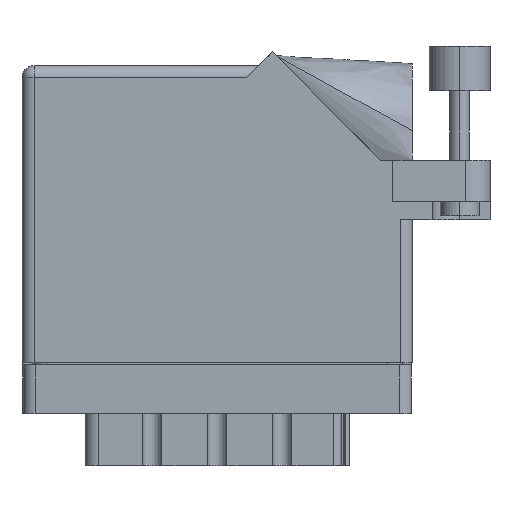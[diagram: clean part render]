
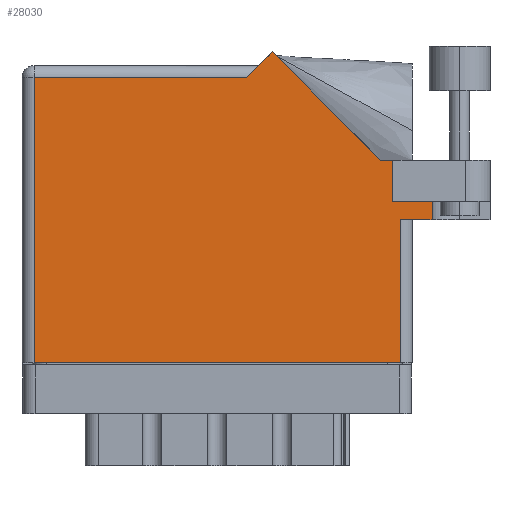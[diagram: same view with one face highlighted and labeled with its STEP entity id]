
A CAD part, front view. The second image highlights one B-rep face of the part: STEP entity #28030.
In plain terms, the highlighted face is planar.
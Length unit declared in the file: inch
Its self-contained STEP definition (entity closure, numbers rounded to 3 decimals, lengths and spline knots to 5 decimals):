
#118 = DIRECTION ( 'NONE',  ( -1., 0., 0. ) ) ;
#1731 = VERTEX_POINT ( 'NONE', #14661 ) ;
#2083 = EDGE_CURVE ( 'NONE', #19479, #13352, #11868, .T. ) ;
#2541 = DIRECTION ( 'NONE',  ( 1., 0., 0. ) ) ;
#3528 = VERTEX_POINT ( 'NONE', #22931 ) ;
#3869 = VERTEX_POINT ( 'NONE', #12422 ) ;
#3912 = CARTESIAN_POINT ( 'NONE',  ( 1.84442, 1.044, 0. ) ) ;
#4193 = VECTOR ( 'NONE', #34545, 39.37008 ) ;
#4266 = DIRECTION ( 'NONE',  ( 0., -1., 0. ) ) ;
#4327 = CARTESIAN_POINT ( 'NONE',  ( 1.91, 1.044, 0. ) ) ;
#4435 = EDGE_CURVE ( 'NONE', #34579, #14940, #30668, .T. ) ;
#4520 = EDGE_LOOP ( 'NONE', ( #21431, #22814, #37123, #25064, #10569, #27595, #11971, #12801, #34658, #15115, #20238 ) ) ;
#4887 = LINE ( 'NONE', #36116, #20215 ) ;
#4944 = CARTESIAN_POINT ( 'NONE',  ( 1.948, 0.737, 0. ) ) ;
#5137 = VERTEX_POINT ( 'NONE', #13821 ) ;
#6867 = DIRECTION ( 'NONE',  ( 1., 0., 0. ) ) ;
#7473 = VECTOR ( 'NONE', #18534, 39.37008 ) ;
#7960 = LINE ( 'NONE', #20940, #7473 ) ;
#8354 = CARTESIAN_POINT ( 'NONE',  ( 0., 0., 0. ) ) ;
#9643 = DIRECTION ( 'NONE',  ( -1., 0., 0. ) ) ;
#9799 = VERTEX_POINT ( 'NONE', #17633 ) ;
#10569 = ORIENTED_EDGE ( 'NONE', *, *, #37462, .F. ) ;
#11868 = LINE ( 'NONE', #25156, #4193 ) ;
#11971 = ORIENTED_EDGE ( 'NONE', *, *, #4435, .T. ) ;
#12422 = CARTESIAN_POINT ( 'NONE',  ( 0.062, 1.468, 0. ) ) ;
#12801 = ORIENTED_EDGE ( 'NONE', *, *, #26107, .T. ) ;
#13094 = DIRECTION ( 'NONE',  ( -1., 0., 0. ) ) ;
#13183 = VECTOR ( 'NONE', #6867, 39.37008 ) ;
#13352 = VERTEX_POINT ( 'NONE', #13732 ) ;
#13732 = CARTESIAN_POINT ( 'NONE',  ( 1.155, 1.468, 0. ) ) ;
#13821 = CARTESIAN_POINT ( 'NONE',  ( 2.1115, 0.831, 0. ) ) ;
#13964 = VERTEX_POINT ( 'NONE', #18599 ) ;
#14661 = CARTESIAN_POINT ( 'NONE',  ( 1.948, 0., 0. ) ) ;
#14867 = CARTESIAN_POINT ( 'NONE',  ( 0., 1.53, 0. ) ) ;
#14940 = VERTEX_POINT ( 'NONE', #3912 ) ;
#15115 = ORIENTED_EDGE ( 'NONE', *, *, #18974, .T. ) ;
#16641 = VERTEX_POINT ( 'NONE', #19869 ) ;
#17633 = CARTESIAN_POINT ( 'NONE',  ( 0.062, 0., 0. ) ) ;
#18131 = LINE ( 'NONE', #27592, #13183 ) ;
#18180 = VECTOR ( 'NONE', #118, 39.37008 ) ;
#18534 = DIRECTION ( 'NONE',  ( 0., -1., 0. ) ) ;
#18599 = CARTESIAN_POINT ( 'NONE',  ( 1.91, 0.831, 0. ) ) ;
#18913 = CARTESIAN_POINT ( 'NONE',  ( 1.84442, 1.044, 0. ) ) ;
#18974 = EDGE_CURVE ( 'NONE', #13352, #3869, #25906, .T. ) ;
#19479 = VERTEX_POINT ( 'NONE', #35683 ) ;
#19869 = CARTESIAN_POINT ( 'NONE',  ( 2.1115, 0.737, 0. ) ) ;
#20206 = EDGE_CURVE ( 'NONE', #3869, #9799, #24911, .T. ) ;
#20215 = VECTOR ( 'NONE', #21914, 39.37008 ) ;
#20238 = ORIENTED_EDGE ( 'NONE', *, *, #20206, .T. ) ;
#20940 = CARTESIAN_POINT ( 'NONE',  ( 2.1115, 1.16177, 0. ) ) ;
#21431 = ORIENTED_EDGE ( 'NONE', *, *, #36397, .T. ) ;
#21506 = EDGE_CURVE ( 'NONE', #1731, #3528, #32529, .T. ) ;
#21914 = DIRECTION ( 'NONE',  ( 1., 0., 0. ) ) ;
#22581 = LINE ( 'NONE', #18913, #28486 ) ;
#22814 = ORIENTED_EDGE ( 'NONE', *, *, #21506, .T. ) ;
#22931 = CARTESIAN_POINT ( 'NONE',  ( 1.948, 0.737, 0. ) ) ;
#23036 = CARTESIAN_POINT ( 'NONE',  ( 1.91, 0.831, 0. ) ) ;
#23091 = AXIS2_PLACEMENT_3D ( 'NONE', #14867, #35147, #13094 ) ;
#24778 = DIRECTION ( 'NONE',  ( -0.707, 0.707, 0. ) ) ;
#24851 = VECTOR ( 'NONE', #27693, 39.37008 ) ;
#24911 = LINE ( 'NONE', #36129, #34439 ) ;
#25064 = ORIENTED_EDGE ( 'NONE', *, *, #31123, .F. ) ;
#25156 = CARTESIAN_POINT ( 'NONE',  ( 1.217, 1.53, 0. ) ) ;
#25906 = LINE ( 'NONE', #28944, #18180 ) ;
#26107 = EDGE_CURVE ( 'NONE', #14940, #19479, #22581, .T. ) ;
#27592 = CARTESIAN_POINT ( 'NONE',  ( 1.91, 0.831, 0. ) ) ;
#27595 = ORIENTED_EDGE ( 'NONE', *, *, #32107, .T. ) ;
#27693 = DIRECTION ( 'NONE',  ( 0., 1., 0. ) ) ;
#27724 = VECTOR ( 'NONE', #34959, 39.37008 ) ;
#28030 = ADVANCED_FACE ( 'NONE', ( #33804 ), #32216, .F. ) ;
#28486 = VECTOR ( 'NONE', #24778, 39.37008 ) ;
#28852 = VECTOR ( 'NONE', #9643, 39.37008 ) ;
#28944 = CARTESIAN_POINT ( 'NONE',  ( 0., 1.468, 0. ) ) ;
#30173 = LINE ( 'NONE', #8354, #32450 ) ;
#30668 = LINE ( 'NONE', #32541, #28852 ) ;
#31123 = EDGE_CURVE ( 'NONE', #5137, #16641, #7960, .T. ) ;
#32107 = EDGE_CURVE ( 'NONE', #13964, #34579, #34999, .T. ) ;
#32216 = PLANE ( 'NONE',  #23091 ) ;
#32450 = VECTOR ( 'NONE', #2541, 39.37008 ) ;
#32529 = LINE ( 'NONE', #4944, #24851 ) ;
#32541 = CARTESIAN_POINT ( 'NONE',  ( 2.41, 1.044, 0. ) ) ;
#33804 = FACE_OUTER_BOUND ( 'NONE', #4520, .T. ) ;
#34439 = VECTOR ( 'NONE', #4266, 39.37008 ) ;
#34545 = DIRECTION ( 'NONE',  ( -0.707, -0.707, 0. ) ) ;
#34579 = VERTEX_POINT ( 'NONE', #4327 ) ;
#34658 = ORIENTED_EDGE ( 'NONE', *, *, #2083, .T. ) ;
#34959 = DIRECTION ( 'NONE',  ( 0., 1., 0. ) ) ;
#34999 = LINE ( 'NONE', #23036, #27724 ) ;
#35147 = DIRECTION ( 'NONE',  ( 0., 0., -1. ) ) ;
#35683 = CARTESIAN_POINT ( 'NONE',  ( 1.28771, 1.60071, 0. ) ) ;
#35885 = EDGE_CURVE ( 'NONE', #3528, #16641, #4887, .T. ) ;
#36116 = CARTESIAN_POINT ( 'NONE',  ( 2.01, 0.737, 0. ) ) ;
#36129 = CARTESIAN_POINT ( 'NONE',  ( 0.062, 0., 0. ) ) ;
#36397 = EDGE_CURVE ( 'NONE', #9799, #1731, #30173, .T. ) ;
#37123 = ORIENTED_EDGE ( 'NONE', *, *, #35885, .T. ) ;
#37462 = EDGE_CURVE ( 'NONE', #13964, #5137, #18131, .T. ) ;
